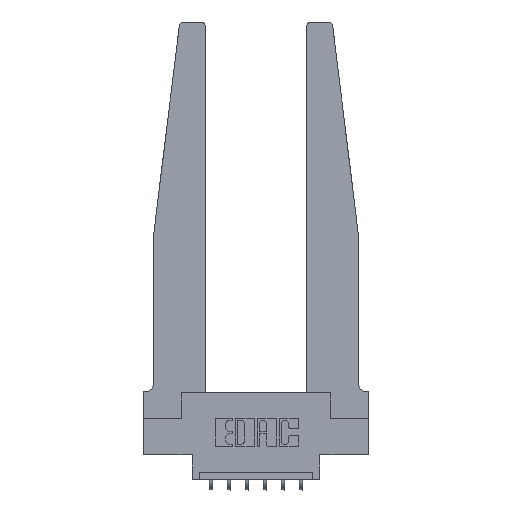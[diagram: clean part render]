
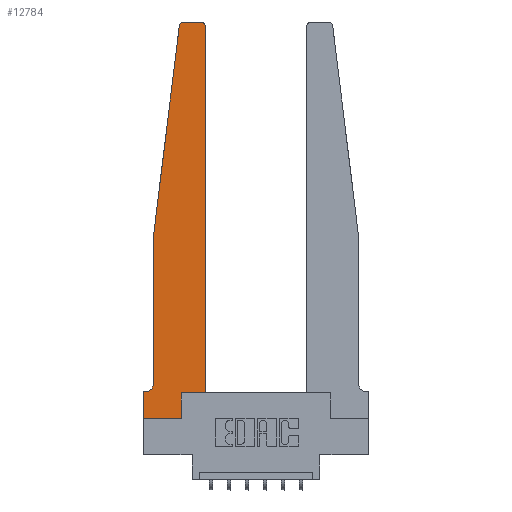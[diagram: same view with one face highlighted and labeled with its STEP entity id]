
A CAD part, top view. The second image highlights one B-rep face of the part: STEP entity #12784.
In plain terms, the highlighted planar face has unit normal (0, 0, 1).
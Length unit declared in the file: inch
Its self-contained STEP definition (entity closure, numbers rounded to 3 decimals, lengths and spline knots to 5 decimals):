
#208 = DIRECTION ( 'NONE',  ( 1., 0., 0. ) ) ;
#379 = AXIS2_PLACEMENT_3D ( 'NONE', #11479, #8124, #8055 ) ;
#434 = DIRECTION ( 'NONE',  ( 0., 1., 0. ) ) ;
#497 = EDGE_LOOP ( 'NONE', ( #1320, #6901, #8226, #8443, #2112, #2566, #8122, #1987, #2368, #9153, #11190, #11829 ) ) ;
#622 = DIRECTION ( 'NONE',  ( 0., -1., 0. ) ) ;
#704 = CARTESIAN_POINT ( 'NONE',  ( 0.065, 0.2375, 0.37 ) ) ;
#776 = CARTESIAN_POINT ( 'NONE',  ( 0.2605, 0., 0.37 ) ) ;
#914 = DIRECTION ( 'NONE',  ( -1., 0., 0. ) ) ;
#1053 = CIRCLE ( 'NONE', #379, 0.03 ) ;
#1295 = LINE ( 'NONE', #5605, #9142 ) ;
#1320 = ORIENTED_EDGE ( 'NONE', *, *, #3182, .T. ) ;
#1393 = EDGE_CURVE ( 'NONE', #7055, #10594, #1295, .T. ) ;
#1573 = PLANE ( 'NONE',  #3478 ) ;
#1680 = EDGE_CURVE ( 'NONE', #4758, #2796, #4197, .T. ) ;
#1987 = ORIENTED_EDGE ( 'NONE', *, *, #8713, .T. ) ;
#2112 = ORIENTED_EDGE ( 'NONE', *, *, #3175, .T. ) ;
#2139 = DIRECTION ( 'NONE',  ( 0., 0., 1. ) ) ;
#2254 = VECTOR ( 'NONE', #13098, 39.37008 ) ;
#2299 = EDGE_CURVE ( 'NONE', #3671, #7055, #1053, .T. ) ;
#2368 = ORIENTED_EDGE ( 'NONE', *, *, #12050, .T. ) ;
#2566 = ORIENTED_EDGE ( 'NONE', *, *, #3448, .T. ) ;
#2594 = LINE ( 'NONE', #11194, #11884 ) ;
#2648 = VECTOR ( 'NONE', #11802, 39.37008 ) ;
#2687 = EDGE_CURVE ( 'NONE', #2796, #7864, #6685, .T. ) ;
#2796 = VERTEX_POINT ( 'NONE', #11744 ) ;
#3175 = EDGE_CURVE ( 'NONE', #11092, #7443, #8260, .T. ) ;
#3182 = EDGE_CURVE ( 'NONE', #7864, #3671, #7197, .T. ) ;
#3448 = EDGE_CURVE ( 'NONE', #7443, #5698, #3825, .T. ) ;
#3478 = AXIS2_PLACEMENT_3D ( 'NONE', #5949, #8983, #8039 ) ;
#3671 = VERTEX_POINT ( 'NONE', #12918 ) ;
#3814 = CARTESIAN_POINT ( 'NONE',  ( 0.395, 2.75, 0.37 ) ) ;
#3825 = LINE ( 'NONE', #8075, #8571 ) ;
#4072 = CARTESIAN_POINT ( 'NONE',  ( 0.395, 2.72, 0.37 ) ) ;
#4197 = LINE ( 'NONE', #9386, #11641 ) ;
#4620 = CARTESIAN_POINT ( 'NONE',  ( 0., 0., 0.37 ) ) ;
#4758 = VERTEX_POINT ( 'NONE', #6370 ) ;
#4796 = CARTESIAN_POINT ( 'NONE',  ( 0.2605, 0.18, 0.37 ) ) ;
#5366 = DIRECTION ( 'NONE',  ( 0., 0., -1. ) ) ;
#5566 = CARTESIAN_POINT ( 'NONE',  ( 0.425, 0.18, 0.37 ) ) ;
#5567 = VECTOR ( 'NONE', #434, 39.37008 ) ;
#5605 = CARTESIAN_POINT ( 'NONE',  ( 0.065, 1.25, 0.37 ) ) ;
#5698 = VERTEX_POINT ( 'NONE', #11752 ) ;
#5949 = CARTESIAN_POINT ( 'NONE',  ( 0., 0.1875, 0.37 ) ) ;
#6132 = VECTOR ( 'NONE', #6888, 39.37008 ) ;
#6370 = CARTESIAN_POINT ( 'NONE',  ( 0.425, 0.18, 0.37 ) ) ;
#6645 = LINE ( 'NONE', #10094, #5567 ) ;
#6685 = CIRCLE ( 'NONE', #9158, 0.03 ) ;
#6821 = LINE ( 'NONE', #8056, #6132 ) ;
#6888 = DIRECTION ( 'NONE',  ( 1., 0., 0. ) ) ;
#6901 = ORIENTED_EDGE ( 'NONE', *, *, #2299, .T. ) ;
#6903 = EDGE_CURVE ( 'NONE', #5698, #8399, #11026, .T. ) ;
#7055 = VERTEX_POINT ( 'NONE', #9252 ) ;
#7197 = LINE ( 'NONE', #13859, #2648 ) ;
#7443 = VERTEX_POINT ( 'NONE', #8956 ) ;
#7640 = VERTEX_POINT ( 'NONE', #776 ) ;
#7825 = EDGE_CURVE ( 'NONE', #10076, #4758, #9856, .T. ) ;
#7864 = VERTEX_POINT ( 'NONE', #3814 ) ;
#8039 = DIRECTION ( 'NONE',  ( 1., 0., 0. ) ) ;
#8055 = DIRECTION ( 'NONE',  ( 1., 0., 0. ) ) ;
#8056 = CARTESIAN_POINT ( 'NONE',  ( 0., 0., 0.37 ) ) ;
#8075 = CARTESIAN_POINT ( 'NONE',  ( 0.065, 0.1875, 0.37 ) ) ;
#8122 = ORIENTED_EDGE ( 'NONE', *, *, #6903, .T. ) ;
#8124 = DIRECTION ( 'NONE',  ( 0., 0., 1. ) ) ;
#8226 = ORIENTED_EDGE ( 'NONE', *, *, #1393, .T. ) ;
#8260 = CIRCLE ( 'NONE', #13712, 0.05 ) ;
#8399 = VERTEX_POINT ( 'NONE', #11439 ) ;
#8443 = ORIENTED_EDGE ( 'NONE', *, *, #11469, .T. ) ;
#8571 = VECTOR ( 'NONE', #13287, 39.37008 ) ;
#8713 = EDGE_CURVE ( 'NONE', #8399, #7640, #6821, .T. ) ;
#8956 = CARTESIAN_POINT ( 'NONE',  ( 0.015, 0.1875, 0.37 ) ) ;
#8983 = DIRECTION ( 'NONE',  ( 0., 0., 1. ) ) ;
#9142 = VECTOR ( 'NONE', #11905, 39.37008 ) ;
#9153 = ORIENTED_EDGE ( 'NONE', *, *, #7825, .T. ) ;
#9158 = AXIS2_PLACEMENT_3D ( 'NONE', #4072, #2139, #12743 ) ;
#9252 = CARTESIAN_POINT ( 'NONE',  ( 0.24675, 2.72367, 0.37 ) ) ;
#9386 = CARTESIAN_POINT ( 'NONE',  ( 0.425, 0.18, 0.37 ) ) ;
#9856 = LINE ( 'NONE', #5566, #10174 ) ;
#10076 = VERTEX_POINT ( 'NONE', #4796 ) ;
#10094 = CARTESIAN_POINT ( 'NONE',  ( 0.2605, 0.18, 0.37 ) ) ;
#10173 = CARTESIAN_POINT ( 'NONE',  ( 0.065, 1.25, 0.37 ) ) ;
#10174 = VECTOR ( 'NONE', #208, 39.37008 ) ;
#10566 = CARTESIAN_POINT ( 'NONE',  ( 0.015, 0.2375, 0.37 ) ) ;
#10594 = VERTEX_POINT ( 'NONE', #10173 ) ;
#11026 = LINE ( 'NONE', #4620, #2254 ) ;
#11092 = VERTEX_POINT ( 'NONE', #704 ) ;
#11190 = ORIENTED_EDGE ( 'NONE', *, *, #1680, .T. ) ;
#11194 = CARTESIAN_POINT ( 'NONE',  ( 0.065, 1.25, 0.37 ) ) ;
#11439 = CARTESIAN_POINT ( 'NONE',  ( 0., 0., 0.37 ) ) ;
#11469 = EDGE_CURVE ( 'NONE', #10594, #11092, #2594, .T. ) ;
#11479 = CARTESIAN_POINT ( 'NONE',  ( 0.27653, 2.72, 0.37 ) ) ;
#11641 = VECTOR ( 'NONE', #12739, 39.37008 ) ;
#11744 = CARTESIAN_POINT ( 'NONE',  ( 0.425, 2.72, 0.37 ) ) ;
#11752 = CARTESIAN_POINT ( 'NONE',  ( 0., 0.1875, 0.37 ) ) ;
#11802 = DIRECTION ( 'NONE',  ( -1., 0., 0. ) ) ;
#11829 = ORIENTED_EDGE ( 'NONE', *, *, #2687, .T. ) ;
#11884 = VECTOR ( 'NONE', #622, 39.37008 ) ;
#11905 = DIRECTION ( 'NONE',  ( -0.122, -0.992, 0. ) ) ;
#12050 = EDGE_CURVE ( 'NONE', #7640, #10076, #6645, .T. ) ;
#12739 = DIRECTION ( 'NONE',  ( 0., 1., 0. ) ) ;
#12743 = DIRECTION ( 'NONE',  ( 1., 0., 0. ) ) ;
#12784 = ADVANCED_FACE ( 'NONE', ( #13250 ), #1573, .T. ) ;
#12918 = CARTESIAN_POINT ( 'NONE',  ( 0.27653, 2.75, 0.37 ) ) ;
#13098 = DIRECTION ( 'NONE',  ( 0., -1., 0. ) ) ;
#13250 = FACE_OUTER_BOUND ( 'NONE', #497, .T. ) ;
#13287 = DIRECTION ( 'NONE',  ( -1., 0., 0. ) ) ;
#13712 = AXIS2_PLACEMENT_3D ( 'NONE', #10566, #5366, #914 ) ;
#13859 = CARTESIAN_POINT ( 'NONE',  ( 0.25, 2.75, 0.37 ) ) ;
